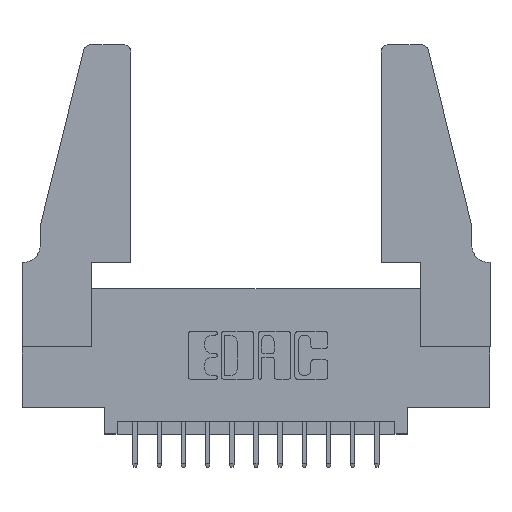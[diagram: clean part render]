
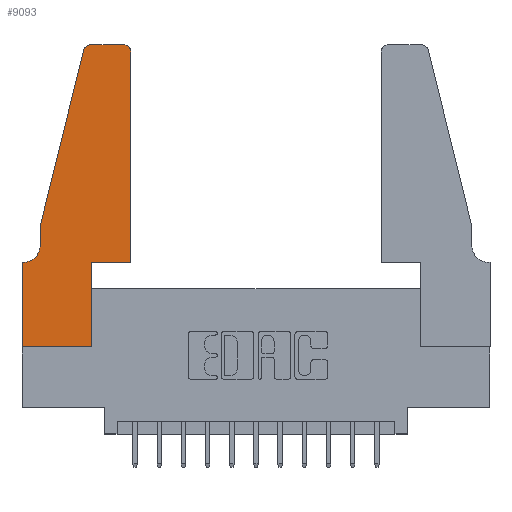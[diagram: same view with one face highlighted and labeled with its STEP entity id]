
A CAD part, top view. The second image highlights one B-rep face of the part: STEP entity #9093.
In plain terms, the highlighted planar face has unit normal (0, 0, 1).
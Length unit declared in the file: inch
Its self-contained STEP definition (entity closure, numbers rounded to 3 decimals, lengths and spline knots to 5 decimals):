
#36 = EDGE_CURVE ( 'NONE', #10202, #4736, #3707, .T. ) ;
#55 = LINE ( 'NONE', #8132, #2180 ) ;
#172 = DIRECTION ( 'NONE',  ( 0., 0., 1. ) ) ;
#503 = VECTOR ( 'NONE', #13253, 39.37008 ) ;
#594 = LINE ( 'NONE', #5308, #13371 ) ;
#847 = CARTESIAN_POINT ( 'NONE',  ( 0.284, 1.25, 0.37 ) ) ;
#855 = CARTESIAN_POINT ( 'NONE',  ( 0., 0., 0.37 ) ) ;
#865 = CARTESIAN_POINT ( 'NONE',  ( 0., 0.35, 0.37 ) ) ;
#991 = ORIENTED_EDGE ( 'NONE', *, *, #6810, .T. ) ;
#1385 = CARTESIAN_POINT ( 'NONE',  ( 0.284, 1.22, 0.37 ) ) ;
#1436 = LINE ( 'NONE', #11815, #7999 ) ;
#1453 = DIRECTION ( 'NONE',  ( -1., 0., 0. ) ) ;
#1549 = VECTOR ( 'NONE', #14956, 39.37008 ) ;
#1557 = ORIENTED_EDGE ( 'NONE', *, *, #5822, .T. ) ;
#1778 = DIRECTION ( 'NONE',  ( 1., 0., 0. ) ) ;
#1817 = CARTESIAN_POINT ( 'NONE',  ( 0.0755, 0.42, 0.37 ) ) ;
#1972 = CIRCLE ( 'NONE', #6930, 0.03 ) ;
#2025 = PLANE ( 'NONE',  #13510 ) ;
#2088 = CARTESIAN_POINT ( 'NONE',  ( 0.4505, 1.22, 0.37 ) ) ;
#2180 = VECTOR ( 'NONE', #4663, 39.37008 ) ;
#2383 = LINE ( 'NONE', #6860, #5200 ) ;
#2506 = ORIENTED_EDGE ( 'NONE', *, *, #36, .T. ) ;
#2604 = ORIENTED_EDGE ( 'NONE', *, *, #11431, .T. ) ;
#2668 = LINE ( 'NONE', #9869, #503 ) ;
#2741 = DIRECTION ( 'NONE',  ( 0., -1., 0. ) ) ;
#2970 = VERTEX_POINT ( 'NONE', #3585 ) ;
#2978 = DIRECTION ( 'NONE',  ( 0., 0., 1. ) ) ;
#3266 = VERTEX_POINT ( 'NONE', #9948 ) ;
#3585 = CARTESIAN_POINT ( 'NONE',  ( 0.2865, 0.35, 0.37 ) ) ;
#3662 = CARTESIAN_POINT ( 'NONE',  ( 0.2865, 0., 0.37 ) ) ;
#3707 = CIRCLE ( 'NONE', #12285, 0.03 ) ;
#3841 = VERTEX_POINT ( 'NONE', #3662 ) ;
#4311 = VERTEX_POINT ( 'NONE', #11507 ) ;
#4347 = CARTESIAN_POINT ( 'NONE',  ( 0.0755, 0.5, 0.37 ) ) ;
#4351 = LINE ( 'NONE', #855, #5241 ) ;
#4355 = VERTEX_POINT ( 'NONE', #14305 ) ;
#4363 = FACE_OUTER_BOUND ( 'NONE', #8667, .T. ) ;
#4466 = ORIENTED_EDGE ( 'NONE', *, *, #4745, .T. ) ;
#4663 = DIRECTION ( 'NONE',  ( 0., -1., 0. ) ) ;
#4736 = VERTEX_POINT ( 'NONE', #10184 ) ;
#4745 = EDGE_CURVE ( 'NONE', #11609, #3841, #4351, .T. ) ;
#4945 = DIRECTION ( 'NONE',  ( -1., 0., 0. ) ) ;
#5095 = CARTESIAN_POINT ( 'NONE',  ( 0.2605, 1.25, 0.37 ) ) ;
#5200 = VECTOR ( 'NONE', #10587, 39.37008 ) ;
#5241 = VECTOR ( 'NONE', #7909, 39.37008 ) ;
#5308 = CARTESIAN_POINT ( 'NONE',  ( 0.0755, 0.35, 0.37 ) ) ;
#5822 = EDGE_CURVE ( 'NONE', #4736, #6526, #10474, .T. ) ;
#6120 = LINE ( 'NONE', #9786, #13919 ) ;
#6270 = ORIENTED_EDGE ( 'NONE', *, *, #9587, .T. ) ;
#6526 = VERTEX_POINT ( 'NONE', #12894 ) ;
#6792 = EDGE_CURVE ( 'NONE', #3266, #10202, #10319, .T. ) ;
#6810 = EDGE_CURVE ( 'NONE', #8802, #14687, #9205, .T. ) ;
#6860 = CARTESIAN_POINT ( 'NONE',  ( 0.2865, 0.35, 0.37 ) ) ;
#6930 = AXIS2_PLACEMENT_3D ( 'NONE', #13478, #2978, #1778 ) ;
#6954 = ORIENTED_EDGE ( 'NONE', *, *, #8785, .T. ) ;
#7011 = VECTOR ( 'NONE', #1453, 39.37008 ) ;
#7578 = ORIENTED_EDGE ( 'NONE', *, *, #12739, .T. ) ;
#7909 = DIRECTION ( 'NONE',  ( 1., 0., 0. ) ) ;
#7999 = VECTOR ( 'NONE', #12983, 39.37008 ) ;
#8132 = CARTESIAN_POINT ( 'NONE',  ( 0., 0., 0.37 ) ) ;
#8419 = DIRECTION ( 'NONE',  ( 1., 0., 0. ) ) ;
#8660 = EDGE_CURVE ( 'NONE', #2970, #4355, #1436, .T. ) ;
#8667 = EDGE_LOOP ( 'NONE', ( #13146, #2506, #1557, #13323, #991, #6954, #7578, #4466, #2604, #13894, #9588, #6270 ) ) ;
#8785 = EDGE_CURVE ( 'NONE', #14687, #4311, #594, .T. ) ;
#8802 = VERTEX_POINT ( 'NONE', #1817 ) ;
#8978 = AXIS2_PLACEMENT_3D ( 'NONE', #9850, #12160, #4945 ) ;
#9093 = ADVANCED_FACE ( 'NONE', ( #4363 ), #2025, .T. ) ;
#9133 = DIRECTION ( 'NONE',  ( 0., 0., 1. ) ) ;
#9205 = CIRCLE ( 'NONE', #8978, 0.07 ) ;
#9587 = EDGE_CURVE ( 'NONE', #10293, #3266, #1972, .T. ) ;
#9588 = ORIENTED_EDGE ( 'NONE', *, *, #12905, .T. ) ;
#9786 = CARTESIAN_POINT ( 'NONE',  ( 0.0755, 0.5, 0.37 ) ) ;
#9850 = CARTESIAN_POINT ( 'NONE',  ( 0.0055, 0.42, 0.37 ) ) ;
#9869 = CARTESIAN_POINT ( 'NONE',  ( 0.4505, 0.35, 0.37 ) ) ;
#9948 = CARTESIAN_POINT ( 'NONE',  ( 0.4205, 1.25, 0.37 ) ) ;
#9979 = DIRECTION ( 'NONE',  ( -1., 0., 0. ) ) ;
#10184 = CARTESIAN_POINT ( 'NONE',  ( 0.25487, 1.22718, 0.37 ) ) ;
#10202 = VERTEX_POINT ( 'NONE', #847 ) ;
#10280 = CARTESIAN_POINT ( 'NONE',  ( 0., 0., 0.37 ) ) ;
#10293 = VERTEX_POINT ( 'NONE', #2088 ) ;
#10319 = LINE ( 'NONE', #5095, #7011 ) ;
#10474 = LINE ( 'NONE', #4347, #1549 ) ;
#10587 = DIRECTION ( 'NONE',  ( 0., 1., 0. ) ) ;
#11431 = EDGE_CURVE ( 'NONE', #3841, #2970, #2383, .T. ) ;
#11507 = CARTESIAN_POINT ( 'NONE',  ( 0., 0.35, 0.37 ) ) ;
#11609 = VERTEX_POINT ( 'NONE', #10280 ) ;
#11815 = CARTESIAN_POINT ( 'NONE',  ( 0.4505, 0.35, 0.37 ) ) ;
#12160 = DIRECTION ( 'NONE',  ( 0., 0., -1. ) ) ;
#12285 = AXIS2_PLACEMENT_3D ( 'NONE', #1385, #172, #8419 ) ;
#12346 = DIRECTION ( 'NONE',  ( 1., 0., 0. ) ) ;
#12739 = EDGE_CURVE ( 'NONE', #4311, #11609, #55, .T. ) ;
#12894 = CARTESIAN_POINT ( 'NONE',  ( 0.0755, 0.5, 0.37 ) ) ;
#12905 = EDGE_CURVE ( 'NONE', #4355, #10293, #2668, .T. ) ;
#12983 = DIRECTION ( 'NONE',  ( 1., 0., 0. ) ) ;
#13146 = ORIENTED_EDGE ( 'NONE', *, *, #6792, .T. ) ;
#13253 = DIRECTION ( 'NONE',  ( 0., 1., 0. ) ) ;
#13323 = ORIENTED_EDGE ( 'NONE', *, *, #14513, .T. ) ;
#13371 = VECTOR ( 'NONE', #9979, 39.37008 ) ;
#13478 = CARTESIAN_POINT ( 'NONE',  ( 0.4205, 1.22, 0.37 ) ) ;
#13510 = AXIS2_PLACEMENT_3D ( 'NONE', #865, #9133, #12346 ) ;
#13860 = CARTESIAN_POINT ( 'NONE',  ( 0.0055, 0.35, 0.37 ) ) ;
#13894 = ORIENTED_EDGE ( 'NONE', *, *, #8660, .T. ) ;
#13919 = VECTOR ( 'NONE', #2741, 39.37008 ) ;
#14305 = CARTESIAN_POINT ( 'NONE',  ( 0.4505, 0.35, 0.37 ) ) ;
#14513 = EDGE_CURVE ( 'NONE', #6526, #8802, #6120, .T. ) ;
#14687 = VERTEX_POINT ( 'NONE', #13860 ) ;
#14956 = DIRECTION ( 'NONE',  ( -0.239, -0.971, 0. ) ) ;
